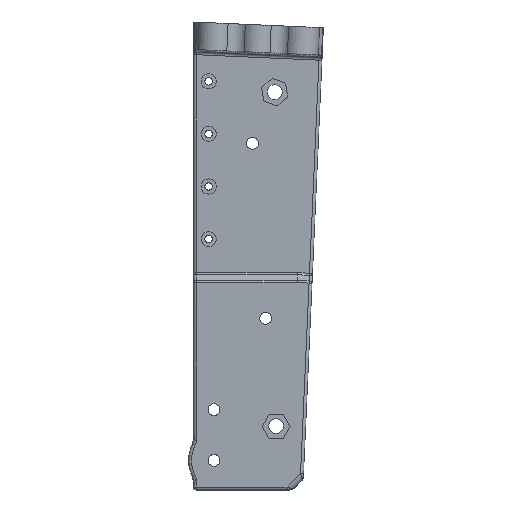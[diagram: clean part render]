
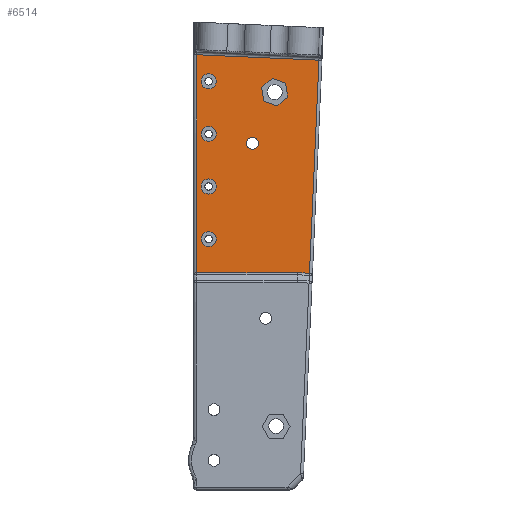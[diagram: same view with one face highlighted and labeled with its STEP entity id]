
A CAD part, left-side view. The second image highlights one B-rep face of the part: STEP entity #6514.
In plain terms, the highlighted planar face has unit normal (-1, 0, 0).
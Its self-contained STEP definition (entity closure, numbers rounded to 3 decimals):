
#342=FACE_BOUND('',#1400,.T.);
#343=FACE_BOUND('',#1401,.T.);
#344=FACE_BOUND('',#1402,.T.);
#345=FACE_BOUND('',#1403,.T.);
#346=FACE_BOUND('',#1404,.T.);
#347=FACE_BOUND('',#1405,.T.);
#401=CIRCLE('',#6712,2.);
#402=CIRCLE('',#6713,2.);
#472=CIRCLE('',#6910,2.54);
#473=CIRCLE('',#6911,2.54);
#477=CIRCLE('',#6917,2.54);
#478=CIRCLE('',#6918,2.54);
#482=CIRCLE('',#6924,2.54);
#483=CIRCLE('',#6925,2.54);
#487=CIRCLE('',#6931,2.54);
#488=CIRCLE('',#6932,2.54);
#687=ELLIPSE('',#7112,2.83,2.);
#976=FACE_OUTER_BOUND('',#1399,.T.);
#1399=EDGE_LOOP('',(#5616,#5617,#5618,#5619,#5620,#5621));
#1400=EDGE_LOOP('',(#5622,#5623,#5624,#5625,#5626,#5627));
#1401=EDGE_LOOP('',(#5628,#5629));
#1402=EDGE_LOOP('',(#5630,#5631));
#1403=EDGE_LOOP('',(#5632,#5633));
#1404=EDGE_LOOP('',(#5634,#5635));
#1405=EDGE_LOOP('',(#5636,#5637));
#1875=LINE('',#11182,#2423);
#1879=LINE('',#11190,#2427);
#1882=LINE('',#11196,#2430);
#1885=LINE('',#11202,#2433);
#1888=LINE('',#11208,#2436);
#1891=LINE('',#11213,#2439);
#1927=LINE('',#11847,#2475);
#1946=LINE('',#12468,#2494);
#1948=LINE('',#12495,#2496);
#1954=LINE('',#12529,#2502);
#1955=LINE('',#12531,#2503);
#2423=VECTOR('',#8164,10.);
#2427=VECTOR('',#8170,10.);
#2430=VECTOR('',#8175,10.);
#2433=VECTOR('',#8180,10.);
#2436=VECTOR('',#8185,10.);
#2439=VECTOR('',#8190,10.);
#2475=VECTOR('',#8508,10.);
#2494=VECTOR('',#8685,10.);
#2496=VECTOR('',#8697,10.);
#2502=VECTOR('',#8717,10.);
#2503=VECTOR('',#8720,10.);
#2800=VERTEX_POINT('',#10137);
#2801=VERTEX_POINT('',#10138);
#2988=VERTEX_POINT('',#11180);
#2989=VERTEX_POINT('',#11181);
#2992=VERTEX_POINT('',#11189);
#2994=VERTEX_POINT('',#11195);
#2996=VERTEX_POINT('',#11201);
#2998=VERTEX_POINT('',#11207);
#3011=VERTEX_POINT('',#11257);
#3012=VERTEX_POINT('',#11259);
#3016=VERTEX_POINT('',#11270);
#3017=VERTEX_POINT('',#11272);
#3021=VERTEX_POINT('',#11283);
#3022=VERTEX_POINT('',#11285);
#3026=VERTEX_POINT('',#11296);
#3027=VERTEX_POINT('',#11298);
#3087=VERTEX_POINT('',#11833);
#3091=VERTEX_POINT('',#11845);
#3154=VERTEX_POINT('',#12461);
#3156=VERTEX_POINT('',#12466);
#3158=VERTEX_POINT('',#12487);
#3160=VERTEX_POINT('',#12493);
#3445=EDGE_CURVE('',#2800,#2801,#401,.T.);
#3446=EDGE_CURVE('',#2801,#2800,#402,.T.);
#3745=EDGE_CURVE('',#2988,#2989,#1875,.T.);
#3749=EDGE_CURVE('',#2992,#2988,#1879,.T.);
#3752=EDGE_CURVE('',#2994,#2992,#1882,.T.);
#3755=EDGE_CURVE('',#2996,#2994,#1885,.T.);
#3758=EDGE_CURVE('',#2998,#2996,#1888,.T.);
#3761=EDGE_CURVE('',#2989,#2998,#1891,.T.);
#3784=EDGE_CURVE('',#3012,#3011,#472,.T.);
#3785=EDGE_CURVE('',#3011,#3012,#473,.T.);
#3790=EDGE_CURVE('',#3017,#3016,#477,.T.);
#3791=EDGE_CURVE('',#3016,#3017,#478,.T.);
#3796=EDGE_CURVE('',#3022,#3021,#482,.T.);
#3797=EDGE_CURVE('',#3021,#3022,#483,.T.);
#3802=EDGE_CURVE('',#3027,#3026,#487,.T.);
#3803=EDGE_CURVE('',#3026,#3027,#488,.T.);
#3901=EDGE_CURVE('',#3091,#3087,#1927,.T.);
#3998=EDGE_CURVE('',#3156,#3154,#1946,.T.);
#4001=EDGE_CURVE('',#3158,#3156,#687,.T.);
#4004=EDGE_CURVE('',#3160,#3158,#1948,.T.);
#4013=EDGE_CURVE('',#3154,#3091,#1954,.T.);
#4014=EDGE_CURVE('',#3087,#3160,#1955,.T.);
#5616=ORIENTED_EDGE('',*,*,#3901,.F.);
#5617=ORIENTED_EDGE('',*,*,#4013,.F.);
#5618=ORIENTED_EDGE('',*,*,#3998,.F.);
#5619=ORIENTED_EDGE('',*,*,#4001,.F.);
#5620=ORIENTED_EDGE('',*,*,#4004,.F.);
#5621=ORIENTED_EDGE('',*,*,#4014,.F.);
#5622=ORIENTED_EDGE('',*,*,#3745,.T.);
#5623=ORIENTED_EDGE('',*,*,#3761,.T.);
#5624=ORIENTED_EDGE('',*,*,#3758,.T.);
#5625=ORIENTED_EDGE('',*,*,#3755,.T.);
#5626=ORIENTED_EDGE('',*,*,#3752,.T.);
#5627=ORIENTED_EDGE('',*,*,#3749,.T.);
#5628=ORIENTED_EDGE('',*,*,#3784,.T.);
#5629=ORIENTED_EDGE('',*,*,#3785,.T.);
#5630=ORIENTED_EDGE('',*,*,#3790,.T.);
#5631=ORIENTED_EDGE('',*,*,#3791,.T.);
#5632=ORIENTED_EDGE('',*,*,#3796,.T.);
#5633=ORIENTED_EDGE('',*,*,#3797,.T.);
#5634=ORIENTED_EDGE('',*,*,#3802,.T.);
#5635=ORIENTED_EDGE('',*,*,#3803,.T.);
#5636=ORIENTED_EDGE('',*,*,#3445,.T.);
#5637=ORIENTED_EDGE('',*,*,#3446,.T.);
#6184=PLANE('',#7160);
#6514=ADVANCED_FACE('',(#976,#342,#343,#344,#345,#346,#347),#6184,.F.);
#6712=AXIS2_PLACEMENT_3D('',#10139,#7611,#7612);
#6713=AXIS2_PLACEMENT_3D('',#10140,#7613,#7614);
#6910=AXIS2_PLACEMENT_3D('',#11260,#8243,#8244);
#6911=AXIS2_PLACEMENT_3D('',#11261,#8245,#8246);
#6917=AXIS2_PLACEMENT_3D('',#11273,#8258,#8259);
#6918=AXIS2_PLACEMENT_3D('',#11274,#8260,#8261);
#6924=AXIS2_PLACEMENT_3D('',#11286,#8273,#8274);
#6925=AXIS2_PLACEMENT_3D('',#11287,#8275,#8276);
#6931=AXIS2_PLACEMENT_3D('',#11299,#8288,#8289);
#6932=AXIS2_PLACEMENT_3D('',#11300,#8290,#8291);
#7112=AXIS2_PLACEMENT_3D('',#12489,#8689,#8690);
#7160=AXIS2_PLACEMENT_3D('',#12670,#8822,#8823);
#7611=DIRECTION('center_axis',(1.,0.,0.));
#7612=DIRECTION('ref_axis',(0.,0.,1.));
#7613=DIRECTION('center_axis',(1.,0.,0.));
#7614=DIRECTION('ref_axis',(0.,0.,1.));
#8164=DIRECTION('',(0.,0.153,0.988));
#8170=DIRECTION('',(0.,0.932,0.362));
#8175=DIRECTION('',(0.,0.78,-0.626));
#8180=DIRECTION('',(0.,-0.153,-0.988));
#8185=DIRECTION('',(0.,-0.932,-0.362));
#8190=DIRECTION('',(0.,-0.78,0.626));
#8243=DIRECTION('center_axis',(1.,0.,0.));
#8244=DIRECTION('ref_axis',(0.,0.,-1.));
#8245=DIRECTION('center_axis',(1.,0.,0.));
#8246=DIRECTION('ref_axis',(0.,0.,-1.));
#8258=DIRECTION('center_axis',(1.,0.,0.));
#8259=DIRECTION('ref_axis',(0.,0.,-1.));
#8260=DIRECTION('center_axis',(1.,0.,0.));
#8261=DIRECTION('ref_axis',(0.,0.,-1.));
#8273=DIRECTION('center_axis',(1.,0.,0.));
#8274=DIRECTION('ref_axis',(0.,0.,-1.));
#8275=DIRECTION('center_axis',(1.,0.,0.));
#8276=DIRECTION('ref_axis',(0.,0.,-1.));
#8288=DIRECTION('center_axis',(1.,0.,0.));
#8289=DIRECTION('ref_axis',(0.,0.,-1.));
#8290=DIRECTION('center_axis',(1.,0.,0.));
#8291=DIRECTION('ref_axis',(0.,0.,-1.));
#8508=DIRECTION('',(0.,-0.999,-0.044));
#8685=DIRECTION('',(0.,1.,0.));
#8689=DIRECTION('center_axis',(-1.,0.,0.));
#8690=DIRECTION('ref_axis',(0.,-0.044,0.999));
#8697=DIRECTION('',(0.,0.999,0.044));
#8717=DIRECTION('',(0.,0.,1.));
#8720=DIRECTION('',(0.,0.044,-0.999));
#8822=DIRECTION('center_axis',(1.,0.,0.));
#8823=DIRECTION('ref_axis',(0.,0.,-1.));
#10137=CARTESIAN_POINT('',(-27.1,-20.,115.2));
#10138=CARTESIAN_POINT('',(-27.1,-20.,119.2));
#10139=CARTESIAN_POINT('Origin',(-27.1,-20.,117.2));
#10140=CARTESIAN_POINT('Origin',(-27.1,-20.,117.2));
#11180=CARTESIAN_POINT('',(-27.1,-23.81,131.535));
#11181=CARTESIAN_POINT('',(-27.1,-23.087,136.213));
#11182=CARTESIAN_POINT('',(-27.1,-25.29,121.957));
#11189=CARTESIAN_POINT('',(-27.1,-28.223,129.821));
#11190=CARTESIAN_POINT('',(-27.1,-28.595,129.677));
#11195=CARTESIAN_POINT('',(-27.1,-31.913,132.787));
#11196=CARTESIAN_POINT('',(-27.1,-23.748,126.225));
#11201=CARTESIAN_POINT('',(-27.1,-31.19,137.465));
#11202=CARTESIAN_POINT('',(-27.1,-33.032,125.548));
#11207=CARTESIAN_POINT('',(-27.1,-26.777,139.179));
#11208=CARTESIAN_POINT('',(-27.1,-29.356,138.178));
#11213=CARTESIAN_POINT('',(-27.1,-16.766,131.134));
#11257=CARTESIAN_POINT('',(-27.1,-5.186,105.126));
#11259=CARTESIAN_POINT('',(-27.1,-5.186,100.046));
#11260=CARTESIAN_POINT('Origin',(-27.1,-5.186,102.586));
#11261=CARTESIAN_POINT('Origin',(-27.1,-5.186,102.586));
#11270=CARTESIAN_POINT('',(-27.1,-5.186,122.906));
#11272=CARTESIAN_POINT('',(-27.1,-5.186,117.826));
#11273=CARTESIAN_POINT('Origin',(-27.1,-5.186,120.366));
#11274=CARTESIAN_POINT('Origin',(-27.1,-5.186,120.366));
#11283=CARTESIAN_POINT('',(-27.1,-5.186,87.346));
#11285=CARTESIAN_POINT('',(-27.1,-5.186,82.266));
#11286=CARTESIAN_POINT('Origin',(-27.1,-5.186,84.806));
#11287=CARTESIAN_POINT('Origin',(-27.1,-5.186,84.806));
#11296=CARTESIAN_POINT('',(-27.1,-5.186,140.686));
#11298=CARTESIAN_POINT('',(-27.1,-5.186,135.606));
#11299=CARTESIAN_POINT('Origin',(-27.1,-5.186,138.146));
#11300=CARTESIAN_POINT('Origin',(-27.1,-5.186,138.146));
#11833=CARTESIAN_POINT('',(-27.1,-42.475,145.293));
#11845=CARTESIAN_POINT('',(-27.1,-1.086,147.136));
#11847=CARTESIAN_POINT('',(-27.1,-22.548,146.181));
#12461=CARTESIAN_POINT('',(-27.1,-1.086,73.456));
#12466=CARTESIAN_POINT('',(-27.1,-35.224,73.456));
#12468=CARTESIAN_POINT('',(-27.1,-11.034,73.456));
#12487=CARTESIAN_POINT('',(-27.1,-35.287,73.454));
#12489=CARTESIAN_POINT('Origin',(-27.1,-35.161,70.627));
#12493=CARTESIAN_POINT('',(-27.1,-39.267,73.277));
#12495=CARTESIAN_POINT('',(-27.1,-27.812,73.787));
#12529=CARTESIAN_POINT('',(-27.1,-1.086,55.823));
#12531=CARTESIAN_POINT('',(-27.1,-39.739,83.86));
#12670=CARTESIAN_POINT('Origin',(-27.1,-22.024,111.646));
